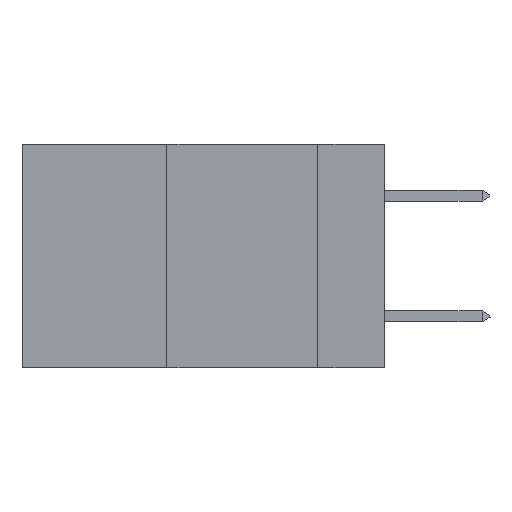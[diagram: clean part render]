
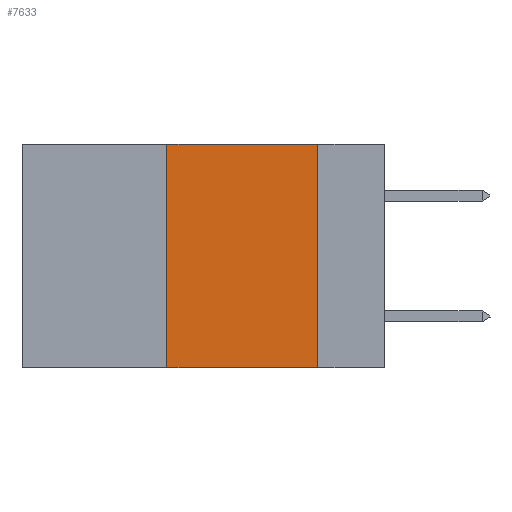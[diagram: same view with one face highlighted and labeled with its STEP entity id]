
A CAD part, left-side view. The second image highlights one B-rep face of the part: STEP entity #7633.
In plain terms, the highlighted planar face has unit normal (-1, 0, 0).
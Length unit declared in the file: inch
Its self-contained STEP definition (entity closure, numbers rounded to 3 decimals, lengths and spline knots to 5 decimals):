
#375 = VERTEX_POINT ( 'NONE', #2544 ) ;
#530 = CARTESIAN_POINT ( 'NONE',  ( 0., 0.11, 0. ) ) ;
#903 = DIRECTION ( 'NONE',  ( 0., -1., 0. ) ) ;
#915 = VERTEX_POINT ( 'NONE', #1344 ) ;
#936 = CARTESIAN_POINT ( 'NONE',  ( 0., 0.11, 0. ) ) ;
#1344 = CARTESIAN_POINT ( 'NONE',  ( 0., 0.36, 0. ) ) ;
#1400 = VECTOR ( 'NONE', #5672, 39.37008 ) ;
#1453 = ORIENTED_EDGE ( 'NONE', *, *, #10357, .F. ) ;
#2262 = DIRECTION ( 'NONE',  ( 0., -1., 0. ) ) ;
#2296 = EDGE_LOOP ( 'NONE', ( #3551, #8605, #1453, #9496 ) ) ;
#2406 = CARTESIAN_POINT ( 'NONE',  ( 0., 0.6, -0.37 ) ) ;
#2544 = CARTESIAN_POINT ( 'NONE',  ( 0., 0.36, -0.37 ) ) ;
#2938 = CARTESIAN_POINT ( 'NONE',  ( 0., 0.6, 0. ) ) ;
#3551 = ORIENTED_EDGE ( 'NONE', *, *, #7847, .F. ) ;
#4503 = LINE ( 'NONE', #7679, #7803 ) ;
#5126 = LINE ( 'NONE', #2406, #5358 ) ;
#5358 = VECTOR ( 'NONE', #903, 39.37008 ) ;
#5364 = DIRECTION ( 'NONE',  ( 0., 0., -1. ) ) ;
#5387 = CARTESIAN_POINT ( 'NONE',  ( 0., 0.11, -0.37 ) ) ;
#5672 = DIRECTION ( 'NONE',  ( 0., 0., -1. ) ) ;
#6169 = PLANE ( 'NONE',  #10241 ) ;
#6177 = DIRECTION ( 'NONE',  ( 0., 0., 1. ) ) ;
#6953 = DIRECTION ( 'NONE',  ( 1., 0., 0. ) ) ;
#6965 = CARTESIAN_POINT ( 'NONE',  ( 0., 0.6, 0. ) ) ;
#7633 = ADVANCED_FACE ( 'NONE', ( #7722 ), #6169, .F. ) ;
#7679 = CARTESIAN_POINT ( 'NONE',  ( 0., 0.36, 0. ) ) ;
#7722 = FACE_OUTER_BOUND ( 'NONE', #2296, .T. ) ;
#7803 = VECTOR ( 'NONE', #6177, 39.37008 ) ;
#7847 = EDGE_CURVE ( 'NONE', #10125, #10013, #8592, .T. ) ;
#8179 = EDGE_CURVE ( 'NONE', #915, #10125, #8198, .T. ) ;
#8198 = LINE ( 'NONE', #6965, #8328 ) ;
#8328 = VECTOR ( 'NONE', #2262, 39.37008 ) ;
#8592 = LINE ( 'NONE', #936, #1400 ) ;
#8605 = ORIENTED_EDGE ( 'NONE', *, *, #8179, .F. ) ;
#8727 = EDGE_CURVE ( 'NONE', #375, #10013, #5126, .T. ) ;
#9496 = ORIENTED_EDGE ( 'NONE', *, *, #8727, .T. ) ;
#10013 = VERTEX_POINT ( 'NONE', #5387 ) ;
#10125 = VERTEX_POINT ( 'NONE', #530 ) ;
#10241 = AXIS2_PLACEMENT_3D ( 'NONE', #2938, #6953, #5364 ) ;
#10357 = EDGE_CURVE ( 'NONE', #375, #915, #4503, .T. ) ;
